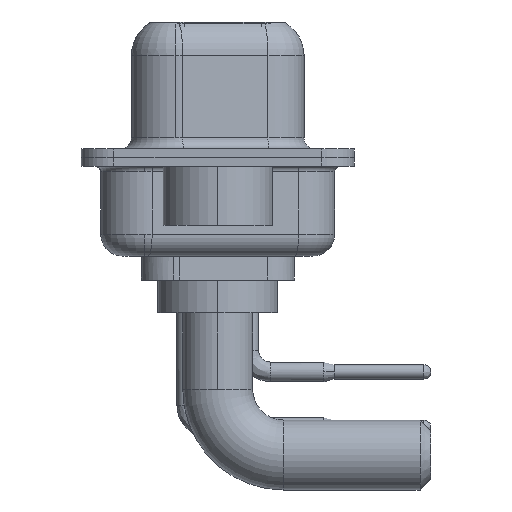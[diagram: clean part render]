
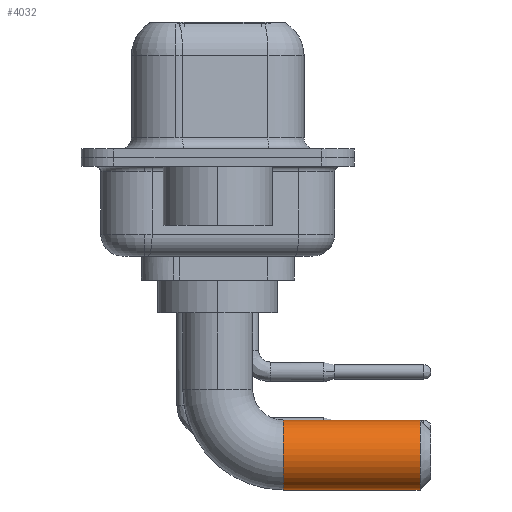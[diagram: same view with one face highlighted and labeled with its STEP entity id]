
A CAD part, left-side view. The second image highlights one B-rep face of the part: STEP entity #4032.
In plain terms, the highlighted cylindrical face has radius 1.6 mm (diameter 3.2 mm), a partial arc.
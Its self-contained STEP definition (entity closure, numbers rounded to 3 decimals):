
#2 = DIRECTION ( 'NONE',  ( 0., 0., -1. ) ) ;
#364 = AXIS2_PLACEMENT_3D ( 'NONE', #8228, #10753, #12234 ) ;
#846 = CARTESIAN_POINT ( 'NONE',  ( 0., -3., -4.9 ) ) ;
#1571 = VERTEX_POINT ( 'NONE', #14077 ) ;
#2516 = CARTESIAN_POINT ( 'NONE',  ( 0., -3., -6.5 ) ) ;
#2675 = EDGE_CURVE ( 'NONE', #6883, #11078, #9219, .T. ) ;
#3717 = CARTESIAN_POINT ( 'NONE',  ( 0., -3., -4.9 ) ) ;
#3991 = ORIENTED_EDGE ( 'NONE', *, *, #2675, .F. ) ;
#4032 = ADVANCED_FACE ( 'NONE', ( #14462 ), #14547, .T. ) ;
#4149 = VERTEX_POINT ( 'NONE', #7929 ) ;
#4591 = DIRECTION ( 'NONE',  ( 0., -1., 0. ) ) ;
#4847 = VECTOR ( 'NONE', #8959, 1000. ) ;
#5021 = DIRECTION ( 'NONE',  ( 0., 1., 0. ) ) ;
#6080 = EDGE_CURVE ( 'NONE', #4149, #11078, #12926, .T. ) ;
#6851 = VECTOR ( 'NONE', #4591, 1000. ) ;
#6883 = VERTEX_POINT ( 'NONE', #846 ) ;
#7251 = EDGE_CURVE ( 'NONE', #1571, #4149, #16435, .T. ) ;
#7838 = DIRECTION ( 'NONE',  ( 0., -1., 0. ) ) ;
#7887 = CIRCLE ( 'NONE', #364, 1.6 ) ;
#7929 = CARTESIAN_POINT ( 'NONE',  ( 0., -9.25, -8.1 ) ) ;
#8228 = CARTESIAN_POINT ( 'NONE',  ( 0., -3., -6.5 ) ) ;
#8342 = CARTESIAN_POINT ( 'NONE',  ( 0., -3., -8.1 ) ) ;
#8823 = AXIS2_PLACEMENT_3D ( 'NONE', #2516, #7838, #2 ) ;
#8959 = DIRECTION ( 'NONE',  ( 0., -1., 0. ) ) ;
#9219 = LINE ( 'NONE', #3717, #4847 ) ;
#10105 = CARTESIAN_POINT ( 'NONE',  ( 0., -9.25, -4.9 ) ) ;
#10331 = CARTESIAN_POINT ( 'NONE',  ( 0., -9.25, -6.5 ) ) ;
#10753 = DIRECTION ( 'NONE',  ( 0., -1., 0. ) ) ;
#11056 = ORIENTED_EDGE ( 'NONE', *, *, #7251, .T. ) ;
#11078 = VERTEX_POINT ( 'NONE', #10105 ) ;
#12234 = DIRECTION ( 'NONE',  ( -1., 0., 0. ) ) ;
#12926 = CIRCLE ( 'NONE', #15717, 1.6 ) ;
#13624 = EDGE_LOOP ( 'NONE', ( #3991, #13670, #11056, #15862 ) ) ;
#13670 = ORIENTED_EDGE ( 'NONE', *, *, #17021, .T. ) ;
#14077 = CARTESIAN_POINT ( 'NONE',  ( 0., -3., -8.1 ) ) ;
#14462 = FACE_OUTER_BOUND ( 'NONE', #13624, .T. ) ;
#14547 = CYLINDRICAL_SURFACE ( 'NONE', #8823, 1.6 ) ;
#15717 = AXIS2_PLACEMENT_3D ( 'NONE', #10331, #5021, #16688 ) ;
#15862 = ORIENTED_EDGE ( 'NONE', *, *, #6080, .T. ) ;
#16435 = LINE ( 'NONE', #8342, #6851 ) ;
#16688 = DIRECTION ( 'NONE',  ( 0., 0., -1. ) ) ;
#17021 = EDGE_CURVE ( 'NONE', #6883, #1571, #7887, .T. ) ;
